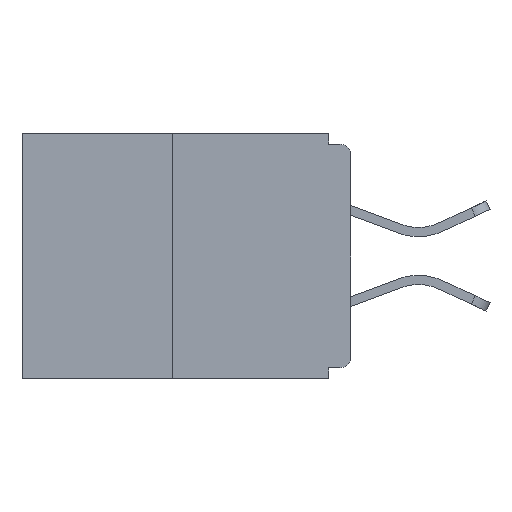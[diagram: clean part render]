
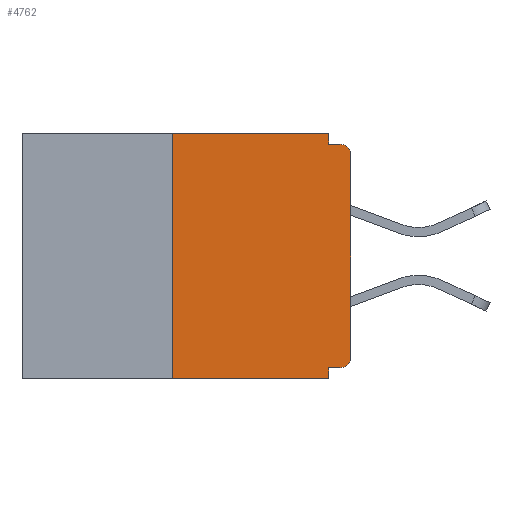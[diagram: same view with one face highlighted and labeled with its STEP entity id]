
A CAD part, left-side view. The second image highlights one B-rep face of the part: STEP entity #4762.
In plain terms, the highlighted planar face has unit normal (-1, 0, 0).
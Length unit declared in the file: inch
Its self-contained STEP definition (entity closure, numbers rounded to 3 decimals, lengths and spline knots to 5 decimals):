
#211 = VECTOR ( 'NONE', #299, 39.37008 ) ;
#251 = VECTOR ( 'NONE', #5719, 39.37008 ) ;
#299 = DIRECTION ( 'NONE',  ( 0., 0., 1. ) ) ;
#543 = VECTOR ( 'NONE', #10209, 39.37008 ) ;
#667 = AXIS2_PLACEMENT_3D ( 'NONE', #16117, #11063, #870 ) ;
#853 = ORIENTED_EDGE ( 'NONE', *, *, #16391, .F. ) ;
#870 = DIRECTION ( 'NONE',  ( 0., 0., -1. ) ) ;
#1327 = LINE ( 'NONE', #12389, #251 ) ;
#1330 = CARTESIAN_POINT ( 'NONE',  ( 0., 0.031, -0.343 ) ) ;
#1416 = ORIENTED_EDGE ( 'NONE', *, *, #9762, .T. ) ;
#1643 = DIRECTION ( 'NONE',  ( 0., -1., 0. ) ) ;
#2034 = EDGE_CURVE ( 'NONE', #7495, #2602, #15630, .T. ) ;
#2463 = CIRCLE ( 'NONE', #10265, 0.015 ) ;
#2602 = VERTEX_POINT ( 'NONE', #14067 ) ;
#2709 = VERTEX_POINT ( 'NONE', #8389 ) ;
#3675 = CARTESIAN_POINT ( 'NONE',  ( 0., 0.46, 0. ) ) ;
#4383 = EDGE_CURVE ( 'NONE', #2709, #18754, #18678, .T. ) ;
#4619 = ORIENTED_EDGE ( 'NONE', *, *, #6029, .T. ) ;
#4698 = CARTESIAN_POINT ( 'NONE',  ( 0., 0.015, -0.015 ) ) ;
#4762 = ADVANCED_FACE ( 'NONE', ( #10885 ), #15792, .F. ) ;
#4842 = CARTESIAN_POINT ( 'NONE',  ( 0., 0., -0.015 ) ) ;
#5668 = LINE ( 'NONE', #4842, #18764 ) ;
#5719 = DIRECTION ( 'NONE',  ( 0., -1., 0. ) ) ;
#6029 = EDGE_CURVE ( 'NONE', #18206, #21952, #22090, .T. ) ;
#7231 = DIRECTION ( 'NONE',  ( 0., 0., -1. ) ) ;
#7327 = ORIENTED_EDGE ( 'NONE', *, *, #14915, .F. ) ;
#7495 = VERTEX_POINT ( 'NONE', #8105 ) ;
#7590 = CARTESIAN_POINT ( 'NONE',  ( 0., 0.031, -0.343 ) ) ;
#8031 = ORIENTED_EDGE ( 'NONE', *, *, #19182, .F. ) ;
#8105 = CARTESIAN_POINT ( 'NONE',  ( 0., 0.031, 0. ) ) ;
#8389 = CARTESIAN_POINT ( 'NONE',  ( 0., 0.25, -0.343 ) ) ;
#8409 = CARTESIAN_POINT ( 'NONE',  ( 0., 0.015, -0.328 ) ) ;
#8677 = DIRECTION ( 'NONE',  ( 0., 0., -1. ) ) ;
#8804 = CARTESIAN_POINT ( 'NONE',  ( 0., 0.46, -0.343 ) ) ;
#8889 = CARTESIAN_POINT ( 'NONE',  ( 0., 0.015, -0.03 ) ) ;
#9345 = CARTESIAN_POINT ( 'NONE',  ( 0., 0., -0.03 ) ) ;
#9674 = EDGE_LOOP ( 'NONE', ( #7327, #21678, #1416, #853, #8031, #17644, #4619, #9881, #19981, #20572 ) ) ;
#9762 = EDGE_CURVE ( 'NONE', #2709, #18055, #17467, .T. ) ;
#9787 = CARTESIAN_POINT ( 'NONE',  ( 0., 0.031, -0.328 ) ) ;
#9881 = ORIENTED_EDGE ( 'NONE', *, *, #15923, .T. ) ;
#10209 = DIRECTION ( 'NONE',  ( 0., 0., 1. ) ) ;
#10265 = AXIS2_PLACEMENT_3D ( 'NONE', #8889, #17160, #8677 ) ;
#10310 = DIRECTION ( 'NONE',  ( 0., 0., -1. ) ) ;
#10704 = LINE ( 'NONE', #7590, #15756 ) ;
#10885 = FACE_OUTER_BOUND ( 'NONE', #9674, .T. ) ;
#11063 = DIRECTION ( 'NONE',  ( -1., 0., 0. ) ) ;
#11839 = VECTOR ( 'NONE', #20759, 39.37008 ) ;
#12119 = CARTESIAN_POINT ( 'NONE',  ( 0., 0.031, 0. ) ) ;
#12389 = CARTESIAN_POINT ( 'NONE',  ( 0., 0.46, 0. ) ) ;
#13373 = CARTESIAN_POINT ( 'NONE',  ( 0., 0., -0.328 ) ) ;
#14067 = CARTESIAN_POINT ( 'NONE',  ( 0., 0.031, -0.015 ) ) ;
#14448 = EDGE_CURVE ( 'NONE', #18663, #18206, #15169, .T. ) ;
#14915 = EDGE_CURVE ( 'NONE', #18754, #7495, #1327, .T. ) ;
#15097 = DIRECTION ( 'NONE',  ( 0., 1., 0. ) ) ;
#15169 = CIRCLE ( 'NONE', #667, 0.015 ) ;
#15285 = EDGE_CURVE ( 'NONE', #2602, #16643, #5668, .T. ) ;
#15574 = DIRECTION ( 'NONE',  ( 1., 0., 0. ) ) ;
#15630 = LINE ( 'NONE', #12119, #19385 ) ;
#15756 = VECTOR ( 'NONE', #17638, 39.37008 ) ;
#15792 = PLANE ( 'NONE',  #19492 ) ;
#15923 = EDGE_CURVE ( 'NONE', #21952, #16643, #2463, .T. ) ;
#16053 = LINE ( 'NONE', #13373, #20113 ) ;
#16117 = CARTESIAN_POINT ( 'NONE',  ( 0., 0.015, -0.313 ) ) ;
#16391 = EDGE_CURVE ( 'NONE', #18680, #18055, #10704, .T. ) ;
#16643 = VERTEX_POINT ( 'NONE', #4698 ) ;
#17160 = DIRECTION ( 'NONE',  ( -1., 0., 0. ) ) ;
#17176 = CARTESIAN_POINT ( 'NONE',  ( 0., 0., -0.313 ) ) ;
#17247 = CARTESIAN_POINT ( 'NONE',  ( 0., 0., 0. ) ) ;
#17467 = LINE ( 'NONE', #8804, #11839 ) ;
#17638 = DIRECTION ( 'NONE',  ( 0., 0., -1. ) ) ;
#17644 = ORIENTED_EDGE ( 'NONE', *, *, #14448, .T. ) ;
#18055 = VERTEX_POINT ( 'NONE', #1330 ) ;
#18206 = VERTEX_POINT ( 'NONE', #17176 ) ;
#18208 = CARTESIAN_POINT ( 'NONE',  ( 0., 0.25, 0. ) ) ;
#18663 = VERTEX_POINT ( 'NONE', #8409 ) ;
#18678 = LINE ( 'NONE', #18796, #543 ) ;
#18680 = VERTEX_POINT ( 'NONE', #9787 ) ;
#18754 = VERTEX_POINT ( 'NONE', #18208 ) ;
#18764 = VECTOR ( 'NONE', #1643, 39.37008 ) ;
#18796 = CARTESIAN_POINT ( 'NONE',  ( 0., 0.25, 0. ) ) ;
#19182 = EDGE_CURVE ( 'NONE', #18663, #18680, #16053, .T. ) ;
#19385 = VECTOR ( 'NONE', #10310, 39.37008 ) ;
#19492 = AXIS2_PLACEMENT_3D ( 'NONE', #3675, #15574, #7231 ) ;
#19981 = ORIENTED_EDGE ( 'NONE', *, *, #15285, .F. ) ;
#20113 = VECTOR ( 'NONE', #15097, 39.37008 ) ;
#20572 = ORIENTED_EDGE ( 'NONE', *, *, #2034, .F. ) ;
#20759 = DIRECTION ( 'NONE',  ( 0., -1., 0. ) ) ;
#21678 = ORIENTED_EDGE ( 'NONE', *, *, #4383, .F. ) ;
#21952 = VERTEX_POINT ( 'NONE', #9345 ) ;
#22090 = LINE ( 'NONE', #17247, #211 ) ;
